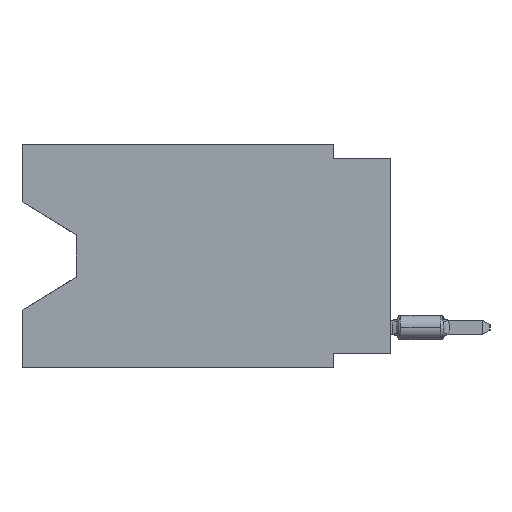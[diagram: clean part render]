
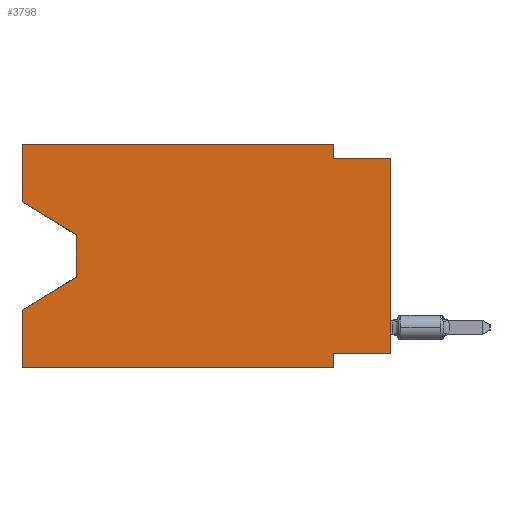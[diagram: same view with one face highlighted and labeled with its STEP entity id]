
A CAD part, left-side view. The second image highlights one B-rep face of the part: STEP entity #3798.
In plain terms, the highlighted planar face has unit normal (-1, 0, 0).
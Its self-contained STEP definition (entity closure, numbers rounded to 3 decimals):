
#147 = CARTESIAN_POINT ( 'NONE',  ( 0., 16.383, 0. ) ) ;
#298 = DIRECTION ( 'NONE',  ( 0., 0., -1. ) ) ;
#448 = FACE_OUTER_BOUND ( 'NONE', #24266, .T. ) ;
#700 = EDGE_CURVE ( 'NONE', #1209, #23666, #28286, .T. ) ;
#869 = ORIENTED_EDGE ( 'NONE', *, *, #15488, .F. ) ;
#1033 = EDGE_CURVE ( 'NONE', #20069, #4528, #29252, .T. ) ;
#1209 = VERTEX_POINT ( 'NONE', #4460 ) ;
#1446 = CARTESIAN_POINT ( 'NONE',  ( 0., 13.97, -4.013 ) ) ;
#1718 = VECTOR ( 'NONE', #13079, 1000. ) ;
#2068 = DIRECTION ( 'NONE',  ( 0., 0.855, -0.519 ) ) ;
#2414 = VERTEX_POINT ( 'NONE', #11445 ) ;
#2873 = CARTESIAN_POINT ( 'NONE',  ( 0., 2.54, -0.635 ) ) ;
#2895 = LINE ( 'NONE', #147, #21443 ) ;
#2950 = CARTESIAN_POINT ( 'NONE',  ( 0., 16.383, 0. ) ) ;
#3147 = CARTESIAN_POINT ( 'NONE',  ( 0., 0., -9.271 ) ) ;
#3798 = ADVANCED_FACE ( 'NONE', ( #448 ), #5450, .F. ) ;
#3885 = CARTESIAN_POINT ( 'NONE',  ( 0., 16.383, -2.546 ) ) ;
#4460 = CARTESIAN_POINT ( 'NONE',  ( 0., 16.383, -9.906 ) ) ;
#4489 = DIRECTION ( 'NONE',  ( 0., 1., 0. ) ) ;
#4528 = VERTEX_POINT ( 'NONE', #2950 ) ;
#4706 = LINE ( 'NONE', #19591, #29384 ) ;
#5243 = ORIENTED_EDGE ( 'NONE', *, *, #29763, .T. ) ;
#5450 = PLANE ( 'NONE',  #31542 ) ;
#5525 = CARTESIAN_POINT ( 'NONE',  ( 0., 2.54, -9.906 ) ) ;
#5875 = ORIENTED_EDGE ( 'NONE', *, *, #18691, .T. ) ;
#5908 = ORIENTED_EDGE ( 'NONE', *, *, #13216, .T. ) ;
#6230 = ORIENTED_EDGE ( 'NONE', *, *, #21238, .F. ) ;
#6307 = DIRECTION ( 'NONE',  ( 0., 0., -1. ) ) ;
#6429 = LINE ( 'NONE', #23908, #6567 ) ;
#6567 = VECTOR ( 'NONE', #11950, 1000. ) ;
#6762 = CARTESIAN_POINT ( 'NONE',  ( 0., 0., -9.271 ) ) ;
#6764 = LINE ( 'NONE', #17115, #10125 ) ;
#7028 = VERTEX_POINT ( 'NONE', #23043 ) ;
#7038 = VERTEX_POINT ( 'NONE', #3147 ) ;
#7152 = VECTOR ( 'NONE', #4489, 1000. ) ;
#7396 = DIRECTION ( 'NONE',  ( 0., 0., 1. ) ) ;
#8268 = LINE ( 'NONE', #15691, #11247 ) ;
#8514 = VECTOR ( 'NONE', #6307, 1000. ) ;
#9458 = VERTEX_POINT ( 'NONE', #2873 ) ;
#9769 = ORIENTED_EDGE ( 'NONE', *, *, #1033, .F. ) ;
#9872 = VERTEX_POINT ( 'NONE', #30814 ) ;
#10125 = VECTOR ( 'NONE', #2068, 1000. ) ;
#10322 = EDGE_CURVE ( 'NONE', #14202, #19643, #18767, .T. ) ;
#10805 = EDGE_CURVE ( 'NONE', #16781, #9458, #12263, .T. ) ;
#11016 = LINE ( 'NONE', #3885, #20095 ) ;
#11247 = VECTOR ( 'NONE', #12793, 1000. ) ;
#11445 = CARTESIAN_POINT ( 'NONE',  ( 0., 2.54, -9.271 ) ) ;
#11890 = VECTOR ( 'NONE', #298, 1000. ) ;
#11950 = DIRECTION ( 'NONE',  ( 0., -1., 0. ) ) ;
#12263 = LINE ( 'NONE', #17119, #23528 ) ;
#12729 = CARTESIAN_POINT ( 'NONE',  ( 0., 16.383, 0. ) ) ;
#12793 = DIRECTION ( 'NONE',  ( 0., -1., 0. ) ) ;
#13079 = DIRECTION ( 'NONE',  ( 0., 0., 1. ) ) ;
#13202 = VECTOR ( 'NONE', #7396, 1000. ) ;
#13216 = EDGE_CURVE ( 'NONE', #7038, #9872, #4706, .T. ) ;
#14171 = EDGE_CURVE ( 'NONE', #2414, #7028, #17827, .T. ) ;
#14202 = VERTEX_POINT ( 'NONE', #29745 ) ;
#14250 = DIRECTION ( 'NONE',  ( 0., 0., 1. ) ) ;
#14706 = CARTESIAN_POINT ( 'NONE',  ( 0., 16.383, -2.546 ) ) ;
#14789 = CARTESIAN_POINT ( 'NONE',  ( 0., 2.54, 0. ) ) ;
#15488 = EDGE_CURVE ( 'NONE', #9458, #9872, #8268, .T. ) ;
#15691 = CARTESIAN_POINT ( 'NONE',  ( 0., 0., -0.635 ) ) ;
#15951 = ORIENTED_EDGE ( 'NONE', *, *, #10805, .F. ) ;
#16318 = EDGE_CURVE ( 'NONE', #7038, #2414, #31512, .T. ) ;
#16781 = VERTEX_POINT ( 'NONE', #14789 ) ;
#17115 = CARTESIAN_POINT ( 'NONE',  ( 0., 13.97, -5.893 ) ) ;
#17119 = CARTESIAN_POINT ( 'NONE',  ( 0., 2.54, 0. ) ) ;
#17508 = CARTESIAN_POINT ( 'NONE',  ( 0., 13.97, -5.893 ) ) ;
#17586 = ORIENTED_EDGE ( 'NONE', *, *, #16318, .F. ) ;
#17827 = LINE ( 'NONE', #5525, #11890 ) ;
#18460 = DIRECTION ( 'NONE',  ( 0., -0.855, -0.519 ) ) ;
#18691 = EDGE_CURVE ( 'NONE', #19643, #23666, #6764, .T. ) ;
#18767 = LINE ( 'NONE', #1446, #8514 ) ;
#19063 = ORIENTED_EDGE ( 'NONE', *, *, #14171, .F. ) ;
#19298 = ORIENTED_EDGE ( 'NONE', *, *, #10322, .T. ) ;
#19591 = CARTESIAN_POINT ( 'NONE',  ( 0., 0., 0. ) ) ;
#19643 = VERTEX_POINT ( 'NONE', #17508 ) ;
#19702 = DIRECTION ( 'NONE',  ( 0., 0., -1. ) ) ;
#20069 = VERTEX_POINT ( 'NONE', #14706 ) ;
#20095 = VECTOR ( 'NONE', #18460, 1000. ) ;
#20192 = DIRECTION ( 'NONE',  ( 1., 0., 0. ) ) ;
#20535 = CARTESIAN_POINT ( 'NONE',  ( 0., 16.383, 0. ) ) ;
#21238 = EDGE_CURVE ( 'NONE', #4528, #16781, #2895, .T. ) ;
#21443 = VECTOR ( 'NONE', #24899, 1000. ) ;
#23043 = CARTESIAN_POINT ( 'NONE',  ( 0., 2.54, -9.906 ) ) ;
#23528 = VECTOR ( 'NONE', #19702, 1000. ) ;
#23666 = VERTEX_POINT ( 'NONE', #27819 ) ;
#23908 = CARTESIAN_POINT ( 'NONE',  ( 0., 16.383, -9.906 ) ) ;
#24266 = EDGE_LOOP ( 'NONE', ( #28896, #19298, #5875, #26687, #5243, #19063, #17586, #5908, #869, #15951, #6230, #9769 ) ) ;
#24899 = DIRECTION ( 'NONE',  ( 0., -1., 0. ) ) ;
#26687 = ORIENTED_EDGE ( 'NONE', *, *, #700, .F. ) ;
#27014 = EDGE_CURVE ( 'NONE', #20069, #14202, #11016, .T. ) ;
#27819 = CARTESIAN_POINT ( 'NONE',  ( 0., 16.383, -7.36 ) ) ;
#28286 = LINE ( 'NONE', #20535, #1718 ) ;
#28896 = ORIENTED_EDGE ( 'NONE', *, *, #27014, .T. ) ;
#29252 = LINE ( 'NONE', #12729, #13202 ) ;
#29384 = VECTOR ( 'NONE', #14250, 1000. ) ;
#29745 = CARTESIAN_POINT ( 'NONE',  ( 0., 13.97, -4.013 ) ) ;
#29763 = EDGE_CURVE ( 'NONE', #1209, #7028, #6429, .T. ) ;
#30052 = DIRECTION ( 'NONE',  ( 0., 0., -1. ) ) ;
#30203 = CARTESIAN_POINT ( 'NONE',  ( 0., 16.383, 0. ) ) ;
#30814 = CARTESIAN_POINT ( 'NONE',  ( 0., 0., -0.635 ) ) ;
#31512 = LINE ( 'NONE', #6762, #7152 ) ;
#31542 = AXIS2_PLACEMENT_3D ( 'NONE', #30203, #20192, #30052 ) ;
